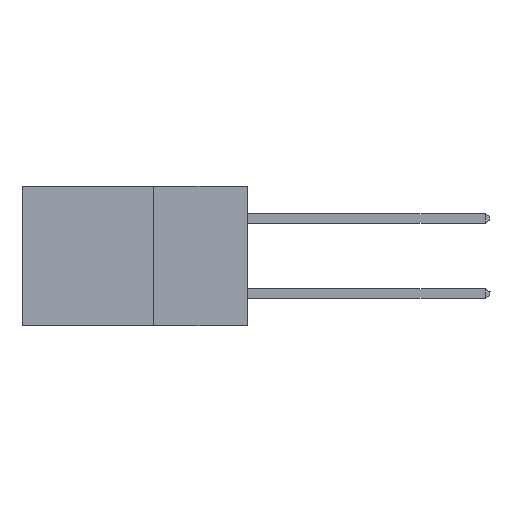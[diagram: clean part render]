
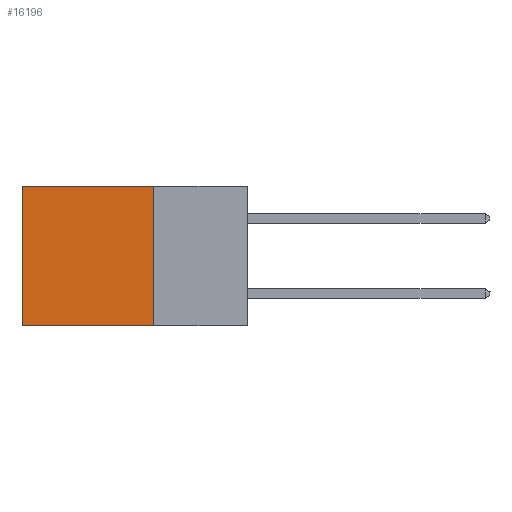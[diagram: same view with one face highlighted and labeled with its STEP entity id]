
A CAD part, left-side view. The second image highlights one B-rep face of the part: STEP entity #16196.
In plain terms, the highlighted planar face has unit normal (-1, 0, 0).
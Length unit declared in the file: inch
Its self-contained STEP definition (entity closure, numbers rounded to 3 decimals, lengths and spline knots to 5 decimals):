
#1053 = EDGE_CURVE ( 'NONE', #18281, #7346, #4565, .T. ) ;
#1088 = EDGE_LOOP ( 'NONE', ( #1908, #11472, #3945, #20889 ) ) ;
#1908 = ORIENTED_EDGE ( 'NONE', *, *, #5518, .T. ) ;
#2123 = LINE ( 'NONE', #2897, #23466 ) ;
#2897 = CARTESIAN_POINT ( 'NONE',  ( 0.298, 0.25, 0. ) ) ;
#3430 = CARTESIAN_POINT ( 'NONE',  ( 0.298, 0.6, -0.37 ) ) ;
#3489 = CARTESIAN_POINT ( 'NONE',  ( 0.298, 0.25, 0. ) ) ;
#3728 = CARTESIAN_POINT ( 'NONE',  ( 0.298, 0.25, 0. ) ) ;
#3945 = ORIENTED_EDGE ( 'NONE', *, *, #22881, .F. ) ;
#3979 = VECTOR ( 'NONE', #21796, 39.37008 ) ;
#4565 = LINE ( 'NONE', #4752, #3979 ) ;
#4752 = CARTESIAN_POINT ( 'NONE',  ( 0.298, 0.25, -0.37 ) ) ;
#5518 = EDGE_CURVE ( 'NONE', #22613, #7346, #22762, .T. ) ;
#5539 = LINE ( 'NONE', #21822, #15209 ) ;
#6777 = CARTESIAN_POINT ( 'NONE',  ( 0.298, 0.6, 0. ) ) ;
#7346 = VERTEX_POINT ( 'NONE', #3430 ) ;
#8108 = VERTEX_POINT ( 'NONE', #3489 ) ;
#11028 = DIRECTION ( 'NONE',  ( 0., 0., -1. ) ) ;
#11472 = ORIENTED_EDGE ( 'NONE', *, *, #1053, .F. ) ;
#12905 = PLANE ( 'NONE',  #17512 ) ;
#15209 = VECTOR ( 'NONE', #16519, 39.37008 ) ;
#15989 = DIRECTION ( 'NONE',  ( 0., 1., 0. ) ) ;
#16196 = ADVANCED_FACE ( 'NONE', ( #21550 ), #12905, .F. ) ;
#16519 = DIRECTION ( 'NONE',  ( 0., 0., -1. ) ) ;
#17272 = CARTESIAN_POINT ( 'NONE',  ( 0.298, 0.6, 0. ) ) ;
#17512 = AXIS2_PLACEMENT_3D ( 'NONE', #3728, #20361, #11028 ) ;
#18074 = CARTESIAN_POINT ( 'NONE',  ( 0.298, 0.25, -0.37 ) ) ;
#18281 = VERTEX_POINT ( 'NONE', #18074 ) ;
#18810 = EDGE_CURVE ( 'NONE', #8108, #22613, #2123, .T. ) ;
#19868 = DIRECTION ( 'NONE',  ( 0., 0., -1. ) ) ;
#20361 = DIRECTION ( 'NONE',  ( 1., 0., 0. ) ) ;
#20889 = ORIENTED_EDGE ( 'NONE', *, *, #18810, .T. ) ;
#21550 = FACE_OUTER_BOUND ( 'NONE', #1088, .T. ) ;
#21796 = DIRECTION ( 'NONE',  ( 0., 1., 0. ) ) ;
#21822 = CARTESIAN_POINT ( 'NONE',  ( 0.298, 0.25, 0. ) ) ;
#22470 = VECTOR ( 'NONE', #19868, 39.37008 ) ;
#22613 = VERTEX_POINT ( 'NONE', #17272 ) ;
#22762 = LINE ( 'NONE', #6777, #22470 ) ;
#22881 = EDGE_CURVE ( 'NONE', #8108, #18281, #5539, .T. ) ;
#23466 = VECTOR ( 'NONE', #15989, 39.37008 ) ;
